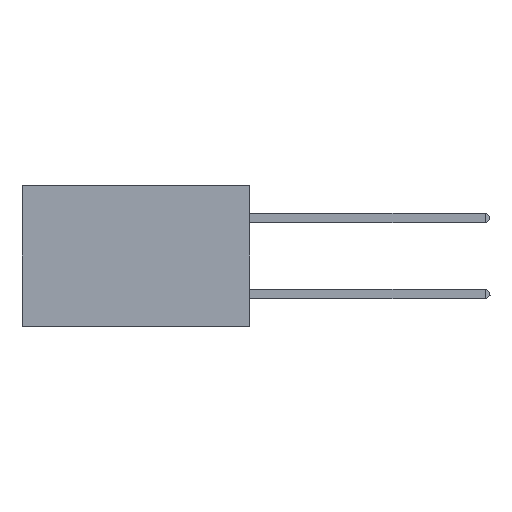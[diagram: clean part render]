
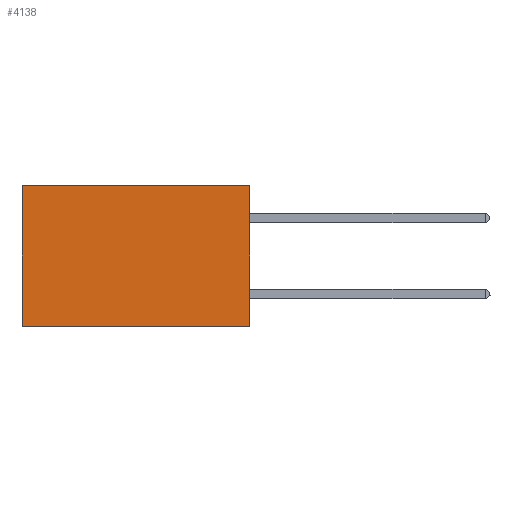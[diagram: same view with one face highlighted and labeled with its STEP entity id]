
A CAD part, left-side view. The second image highlights one B-rep face of the part: STEP entity #4138.
In plain terms, the highlighted planar face has unit normal (-1, 0, 0).
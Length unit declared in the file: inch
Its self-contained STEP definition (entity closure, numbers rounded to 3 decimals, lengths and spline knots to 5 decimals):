
#54 = FACE_OUTER_BOUND ( 'NONE', #18573, .T. ) ;
#514 = VECTOR ( 'NONE', #24520, 39.37008 ) ;
#2628 = ORIENTED_EDGE ( 'NONE', *, *, #11917, .F. ) ;
#3322 = VERTEX_POINT ( 'NONE', #8041 ) ;
#4138 = ADVANCED_FACE ( 'NONE', ( #54 ), #24499, .F. ) ;
#4278 = VECTOR ( 'NONE', #17281, 39.37008 ) ;
#4344 = CARTESIAN_POINT ( 'NONE',  ( 0.2875, 0., 0. ) ) ;
#4591 = CARTESIAN_POINT ( 'NONE',  ( 0.2875, 0., -0.37 ) ) ;
#6868 = DIRECTION ( 'NONE',  ( 0., 0., -1. ) ) ;
#7858 = CARTESIAN_POINT ( 'NONE',  ( 0.2875, 0.6, 0. ) ) ;
#7917 = ORIENTED_EDGE ( 'NONE', *, *, #16471, .T. ) ;
#8041 = CARTESIAN_POINT ( 'NONE',  ( 0.2875, 0., -0.37 ) ) ;
#8251 = DIRECTION ( 'NONE',  ( 0., 1., 0. ) ) ;
#8894 = LINE ( 'NONE', #4344, #17998 ) ;
#9898 = LINE ( 'NONE', #7858, #514 ) ;
#10871 = ORIENTED_EDGE ( 'NONE', *, *, #22223, .F. ) ;
#11890 = CARTESIAN_POINT ( 'NONE',  ( 0.2875, 0.6, 0. ) ) ;
#11917 = EDGE_CURVE ( 'NONE', #3322, #12216, #15392, .T. ) ;
#12216 = VERTEX_POINT ( 'NONE', #20256 ) ;
#12858 = VERTEX_POINT ( 'NONE', #24304 ) ;
#14348 = CARTESIAN_POINT ( 'NONE',  ( 0.2875, 0., 0. ) ) ;
#15392 = LINE ( 'NONE', #4591, #4278 ) ;
#16471 = EDGE_CURVE ( 'NONE', #24674, #12216, #9898, .T. ) ;
#17281 = DIRECTION ( 'NONE',  ( 0., 1., 0. ) ) ;
#17998 = VECTOR ( 'NONE', #8251, 39.37008 ) ;
#18573 = EDGE_LOOP ( 'NONE', ( #7917, #2628, #10871, #24858 ) ) ;
#19515 = EDGE_CURVE ( 'NONE', #12858, #24674, #8894, .T. ) ;
#20256 = CARTESIAN_POINT ( 'NONE',  ( 0.2875, 0.6, -0.37 ) ) ;
#20734 = DIRECTION ( 'NONE',  ( 0., 0., -1. ) ) ;
#21732 = AXIS2_PLACEMENT_3D ( 'NONE', #14348, #24772, #20734 ) ;
#22223 = EDGE_CURVE ( 'NONE', #12858, #3322, #23693, .T. ) ;
#23228 = CARTESIAN_POINT ( 'NONE',  ( 0.2875, 0., 0. ) ) ;
#23693 = LINE ( 'NONE', #23228, #26630 ) ;
#24304 = CARTESIAN_POINT ( 'NONE',  ( 0.2875, 0., 0. ) ) ;
#24499 = PLANE ( 'NONE',  #21732 ) ;
#24520 = DIRECTION ( 'NONE',  ( 0., 0., -1. ) ) ;
#24674 = VERTEX_POINT ( 'NONE', #11890 ) ;
#24772 = DIRECTION ( 'NONE',  ( 1., 0., 0. ) ) ;
#24858 = ORIENTED_EDGE ( 'NONE', *, *, #19515, .T. ) ;
#26630 = VECTOR ( 'NONE', #6868, 39.37008 ) ;
